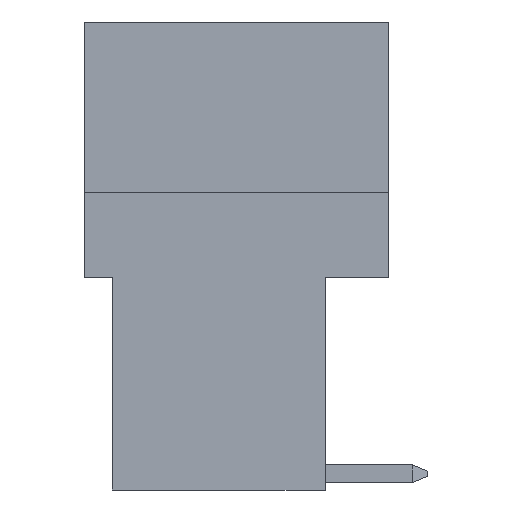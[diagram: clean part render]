
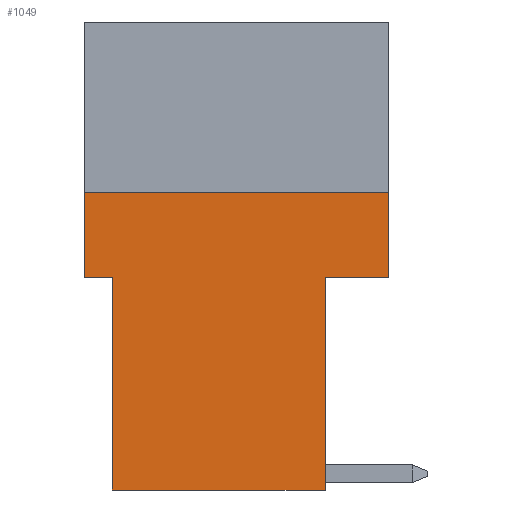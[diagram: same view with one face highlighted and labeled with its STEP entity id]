
A CAD part, left-side view. The second image highlights one B-rep face of the part: STEP entity #1049.
In plain terms, the highlighted planar face has unit normal (-1, 0, 0).
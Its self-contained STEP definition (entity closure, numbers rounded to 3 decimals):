
#2 = EDGE_CURVE ( 'NONE', #426, #9172, #9125, .T. ) ;
#262 = CARTESIAN_POINT ( 'NONE',  ( -47., 4.3, -4.8 ) ) ;
#426 = VERTEX_POINT ( 'NONE', #5687 ) ;
#456 = CARTESIAN_POINT ( 'NONE',  ( -47., 4.3, -13.2 ) ) ;
#602 = CARTESIAN_POINT ( 'NONE',  ( -47., 3.5, -7.2 ) ) ;
#719 = VERTEX_POINT ( 'NONE', #7866 ) ;
#945 = LINE ( 'NONE', #5439, #7199 ) ;
#1042 = DIRECTION ( 'NONE',  ( 0., 1., 0. ) ) ;
#1049 = ADVANCED_FACE ( 'NONE', ( #3301 ), #6710, .T. ) ;
#1084 = VECTOR ( 'NONE', #1663, 1000. ) ;
#1248 = CARTESIAN_POINT ( 'NONE',  ( -47., -2.5, -13.2 ) ) ;
#1385 = EDGE_CURVE ( 'NONE', #719, #7019, #5063, .T. ) ;
#1558 = DIRECTION ( 'NONE',  ( 0., 0., -1. ) ) ;
#1663 = DIRECTION ( 'NONE',  ( 0., 1., 0. ) ) ;
#1812 = CARTESIAN_POINT ( 'NONE',  ( -47., -4.3, -7.2 ) ) ;
#1838 = EDGE_LOOP ( 'NONE', ( #9165, #11097, #8873, #4707, #5609, #7381, #2222, #6872 ) ) ;
#2021 = LINE ( 'NONE', #4689, #10171 ) ;
#2222 = ORIENTED_EDGE ( 'NONE', *, *, #11426, .T. ) ;
#2358 = VECTOR ( 'NONE', #1558, 1000. ) ;
#2523 = VECTOR ( 'NONE', #8406, 1000. ) ;
#2928 = LINE ( 'NONE', #4637, #11254 ) ;
#3010 = AXIS2_PLACEMENT_3D ( 'NONE', #456, #4250, #10309 ) ;
#3172 = EDGE_CURVE ( 'NONE', #9475, #8759, #2928, .T. ) ;
#3301 = FACE_OUTER_BOUND ( 'NONE', #1838, .T. ) ;
#3363 = VECTOR ( 'NONE', #8648, 1000. ) ;
#3463 = CARTESIAN_POINT ( 'NONE',  ( -47., 4.3, -4.8 ) ) ;
#3555 = CARTESIAN_POINT ( 'NONE',  ( -47., -2.5, -7.2 ) ) ;
#3857 = EDGE_CURVE ( 'NONE', #9475, #719, #8915, .T. ) ;
#4250 = DIRECTION ( 'NONE',  ( -1., 0., 0. ) ) ;
#4637 = CARTESIAN_POINT ( 'NONE',  ( -47., -4.3, -13.2 ) ) ;
#4689 = CARTESIAN_POINT ( 'NONE',  ( -47., 4.3, -13.2 ) ) ;
#4707 = ORIENTED_EDGE ( 'NONE', *, *, #6421, .F. ) ;
#4763 = LINE ( 'NONE', #262, #2523 ) ;
#4769 = CARTESIAN_POINT ( 'NONE',  ( -47., 4.3, -7.2 ) ) ;
#5063 = LINE ( 'NONE', #10298, #3363 ) ;
#5099 = LINE ( 'NONE', #602, #2358 ) ;
#5439 = CARTESIAN_POINT ( 'NONE',  ( -47., 4.3, -13.2 ) ) ;
#5493 = DIRECTION ( 'NONE',  ( 0., -1., 0. ) ) ;
#5609 = ORIENTED_EDGE ( 'NONE', *, *, #8189, .F. ) ;
#5687 = CARTESIAN_POINT ( 'NONE',  ( -47., 3.5, -7.2 ) ) ;
#5835 = CARTESIAN_POINT ( 'NONE',  ( -47., -4.3, -4.8 ) ) ;
#6421 = EDGE_CURVE ( 'NONE', #8124, #8759, #4763, .T. ) ;
#6710 = PLANE ( 'NONE',  #3010 ) ;
#6872 = ORIENTED_EDGE ( 'NONE', *, *, #10420, .T. ) ;
#7019 = VERTEX_POINT ( 'NONE', #1248 ) ;
#7199 = VECTOR ( 'NONE', #5493, 1000. ) ;
#7381 = ORIENTED_EDGE ( 'NONE', *, *, #2, .F. ) ;
#7866 = CARTESIAN_POINT ( 'NONE',  ( -47., -2.5, -7.2 ) ) ;
#8124 = VERTEX_POINT ( 'NONE', #3463 ) ;
#8165 = DIRECTION ( 'NONE',  ( 0., 0., 1. ) ) ;
#8189 = EDGE_CURVE ( 'NONE', #9172, #8124, #2021, .T. ) ;
#8406 = DIRECTION ( 'NONE',  ( 0., -1., 0. ) ) ;
#8648 = DIRECTION ( 'NONE',  ( 0., 0., -1. ) ) ;
#8759 = VERTEX_POINT ( 'NONE', #5835 ) ;
#8873 = ORIENTED_EDGE ( 'NONE', *, *, #3172, .T. ) ;
#8898 = CARTESIAN_POINT ( 'NONE',  ( -47., 3.5, -13.2 ) ) ;
#8915 = LINE ( 'NONE', #3555, #1084 ) ;
#9125 = LINE ( 'NONE', #4769, #11273 ) ;
#9165 = ORIENTED_EDGE ( 'NONE', *, *, #1385, .F. ) ;
#9172 = VERTEX_POINT ( 'NONE', #10303 ) ;
#9289 = DIRECTION ( 'NONE',  ( 0., 0., 1. ) ) ;
#9475 = VERTEX_POINT ( 'NONE', #1812 ) ;
#10171 = VECTOR ( 'NONE', #8165, 1000. ) ;
#10298 = CARTESIAN_POINT ( 'NONE',  ( -47., -2.5, -7.2 ) ) ;
#10303 = CARTESIAN_POINT ( 'NONE',  ( -47., 4.3, -7.2 ) ) ;
#10309 = DIRECTION ( 'NONE',  ( 0., 0., 1. ) ) ;
#10420 = EDGE_CURVE ( 'NONE', #10755, #7019, #945, .T. ) ;
#10755 = VERTEX_POINT ( 'NONE', #8898 ) ;
#11097 = ORIENTED_EDGE ( 'NONE', *, *, #3857, .F. ) ;
#11254 = VECTOR ( 'NONE', #9289, 1000. ) ;
#11273 = VECTOR ( 'NONE', #1042, 1000. ) ;
#11426 = EDGE_CURVE ( 'NONE', #426, #10755, #5099, .T. ) ;
